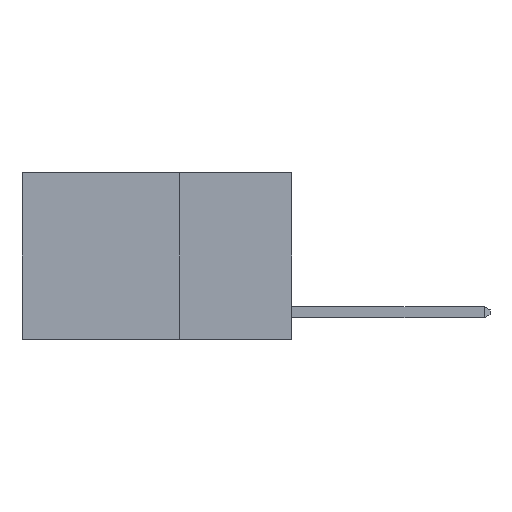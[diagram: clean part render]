
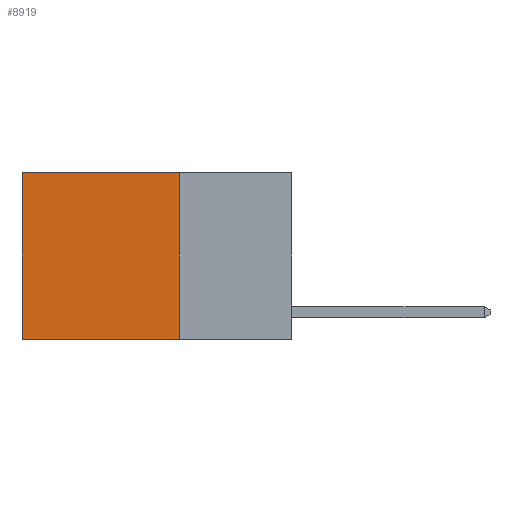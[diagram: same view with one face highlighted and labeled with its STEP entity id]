
A CAD part, left-side view. The second image highlights one B-rep face of the part: STEP entity #8919.
In plain terms, the highlighted planar face has unit normal (-1, 0, 0).
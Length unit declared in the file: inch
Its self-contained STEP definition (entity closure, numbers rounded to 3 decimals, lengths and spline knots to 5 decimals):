
#487 = CARTESIAN_POINT ( 'NONE',  ( 0.2625, 0.6, -0.37 ) ) ;
#607 = LINE ( 'NONE', #7553, #3006 ) ;
#834 = LINE ( 'NONE', #3790, #2941 ) ;
#1192 = DIRECTION ( 'NONE',  ( 0., 0., -1. ) ) ;
#1245 = DIRECTION ( 'NONE',  ( 0., 0., -1. ) ) ;
#1499 = DIRECTION ( 'NONE',  ( 1., 0., 0. ) ) ;
#1663 = CARTESIAN_POINT ( 'NONE',  ( 0.2625, 0.25, 0. ) ) ;
#2103 = CARTESIAN_POINT ( 'NONE',  ( 0.2625, 0.25, 0. ) ) ;
#2626 = FACE_OUTER_BOUND ( 'NONE', #11731, .T. ) ;
#2922 = ORIENTED_EDGE ( 'NONE', *, *, #10982, .F. ) ;
#2941 = VECTOR ( 'NONE', #9210, 39.37008 ) ;
#3006 = VECTOR ( 'NONE', #1192, 39.37008 ) ;
#3027 = EDGE_CURVE ( 'NONE', #6560, #11110, #4281, .T. ) ;
#3514 = AXIS2_PLACEMENT_3D ( 'NONE', #4202, #1499, #7863 ) ;
#3790 = CARTESIAN_POINT ( 'NONE',  ( 0.2625, 0.25, 0. ) ) ;
#4202 = CARTESIAN_POINT ( 'NONE',  ( 0.2625, 0.25, 0. ) ) ;
#4281 = LINE ( 'NONE', #11644, #9103 ) ;
#5326 = DIRECTION ( 'NONE',  ( 0., 1., 0. ) ) ;
#5689 = CARTESIAN_POINT ( 'NONE',  ( 0.2625, 0.25, -0.37 ) ) ;
#6560 = VERTEX_POINT ( 'NONE', #5689 ) ;
#6609 = ORIENTED_EDGE ( 'NONE', *, *, #3027, .F. ) ;
#6849 = VERTEX_POINT ( 'NONE', #7002 ) ;
#7002 = CARTESIAN_POINT ( 'NONE',  ( 0.2625, 0.6, 0. ) ) ;
#7553 = CARTESIAN_POINT ( 'NONE',  ( 0.2625, 0.6, 0. ) ) ;
#7863 = DIRECTION ( 'NONE',  ( 0., 0., -1. ) ) ;
#8027 = EDGE_CURVE ( 'NONE', #8409, #6849, #834, .T. ) ;
#8225 = ORIENTED_EDGE ( 'NONE', *, *, #8027, .T. ) ;
#8257 = LINE ( 'NONE', #2103, #10355 ) ;
#8409 = VERTEX_POINT ( 'NONE', #1663 ) ;
#8919 = ADVANCED_FACE ( 'NONE', ( #2626 ), #11435, .F. ) ;
#9103 = VECTOR ( 'NONE', #5326, 39.37008 ) ;
#9210 = DIRECTION ( 'NONE',  ( 0., 1., 0. ) ) ;
#10205 = ORIENTED_EDGE ( 'NONE', *, *, #11559, .T. ) ;
#10355 = VECTOR ( 'NONE', #1245, 39.37008 ) ;
#10982 = EDGE_CURVE ( 'NONE', #8409, #6560, #8257, .T. ) ;
#11110 = VERTEX_POINT ( 'NONE', #487 ) ;
#11435 = PLANE ( 'NONE',  #3514 ) ;
#11559 = EDGE_CURVE ( 'NONE', #6849, #11110, #607, .T. ) ;
#11644 = CARTESIAN_POINT ( 'NONE',  ( 0.2625, 0.25, -0.37 ) ) ;
#11731 = EDGE_LOOP ( 'NONE', ( #10205, #6609, #2922, #8225 ) ) ;
